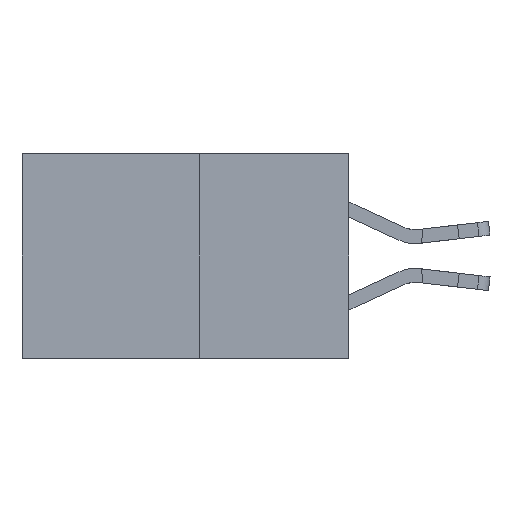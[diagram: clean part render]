
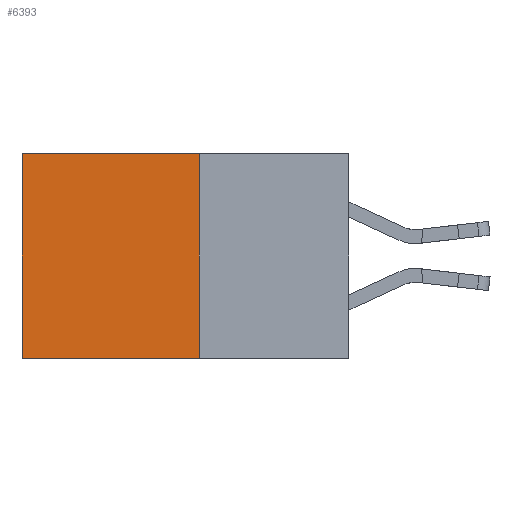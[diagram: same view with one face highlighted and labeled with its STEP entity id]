
A CAD part, left-side view. The second image highlights one B-rep face of the part: STEP entity #6393.
In plain terms, the highlighted planar face has unit normal (-1, 0, 0).
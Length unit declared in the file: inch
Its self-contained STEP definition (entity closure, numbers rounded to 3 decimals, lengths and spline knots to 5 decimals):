
#82 = EDGE_CURVE ( 'NONE', #6809, #7067, #13159, .T. ) ;
#482 = EDGE_CURVE ( 'NONE', #8346, #6809, #3066, .T. ) ;
#1455 = VERTEX_POINT ( 'NONE', #7419 ) ;
#1675 = ORIENTED_EDGE ( 'NONE', *, *, #3353, .F. ) ;
#2157 = ORIENTED_EDGE ( 'NONE', *, *, #482, .T. ) ;
#2599 = VECTOR ( 'NONE', #15812, 39.37008 ) ;
#3066 = LINE ( 'NONE', #16616, #2599 ) ;
#3124 = CARTESIAN_POINT ( 'NONE',  ( 0.277, 0.59, -0.37 ) ) ;
#3353 = EDGE_CURVE ( 'NONE', #8346, #1455, #6255, .T. ) ;
#4126 = AXIS2_PLACEMENT_3D ( 'NONE', #11958, #11937, #11921 ) ;
#4176 = CARTESIAN_POINT ( 'NONE',  ( 0.277, 0.59, 0. ) ) ;
#4342 = ORIENTED_EDGE ( 'NONE', *, *, #82, .T. ) ;
#5216 = CARTESIAN_POINT ( 'NONE',  ( 0.277, 0.27, 0. ) ) ;
#5776 = VECTOR ( 'NONE', #12747, 39.37008 ) ;
#6255 = LINE ( 'NONE', #10754, #5776 ) ;
#6393 = ADVANCED_FACE ( 'NONE', ( #20039 ), #12001, .F. ) ;
#6809 = VERTEX_POINT ( 'NONE', #4176 ) ;
#7067 = VERTEX_POINT ( 'NONE', #17754 ) ;
#7146 = EDGE_CURVE ( 'NONE', #1455, #7067, #11979, .T. ) ;
#7419 = CARTESIAN_POINT ( 'NONE',  ( 0.277, 0.27, -0.37 ) ) ;
#8346 = VERTEX_POINT ( 'NONE', #5216 ) ;
#8723 = DIRECTION ( 'NONE',  ( 0., 0., -1. ) ) ;
#8986 = VECTOR ( 'NONE', #8723, 39.37008 ) ;
#8993 = ORIENTED_EDGE ( 'NONE', *, *, #7146, .F. ) ;
#10108 = DIRECTION ( 'NONE',  ( 0., 1., 0. ) ) ;
#10754 = CARTESIAN_POINT ( 'NONE',  ( 0.277, 0.27, -0.37 ) ) ;
#11921 = DIRECTION ( 'NONE',  ( 0., 0., -1. ) ) ;
#11937 = DIRECTION ( 'NONE',  ( 1., 0., 0. ) ) ;
#11958 = CARTESIAN_POINT ( 'NONE',  ( 0.277, 0.27, -0.37 ) ) ;
#11979 = LINE ( 'NONE', #14821, #15661 ) ;
#12001 = PLANE ( 'NONE',  #4126 ) ;
#12747 = DIRECTION ( 'NONE',  ( 0., 0., -1. ) ) ;
#13159 = LINE ( 'NONE', #3124, #8986 ) ;
#14821 = CARTESIAN_POINT ( 'NONE',  ( 0.277, 0.27, -0.37 ) ) ;
#15661 = VECTOR ( 'NONE', #10108, 39.37008 ) ;
#15812 = DIRECTION ( 'NONE',  ( 0., 1., 0. ) ) ;
#16616 = CARTESIAN_POINT ( 'NONE',  ( 0.277, 0.27, 0. ) ) ;
#17754 = CARTESIAN_POINT ( 'NONE',  ( 0.277, 0.59, -0.37 ) ) ;
#18115 = EDGE_LOOP ( 'NONE', ( #4342, #8993, #1675, #2157 ) ) ;
#20039 = FACE_OUTER_BOUND ( 'NONE', #18115, .T. ) ;
